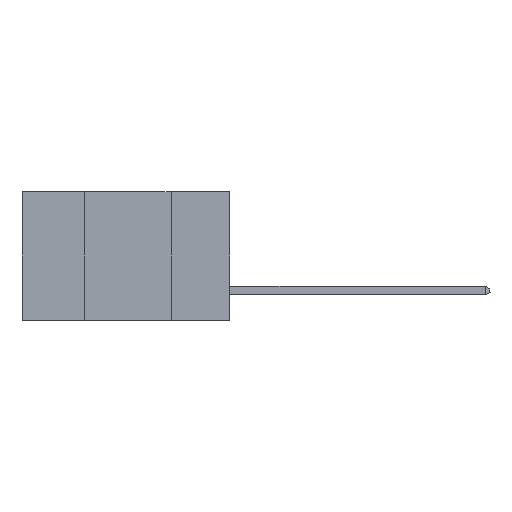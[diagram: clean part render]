
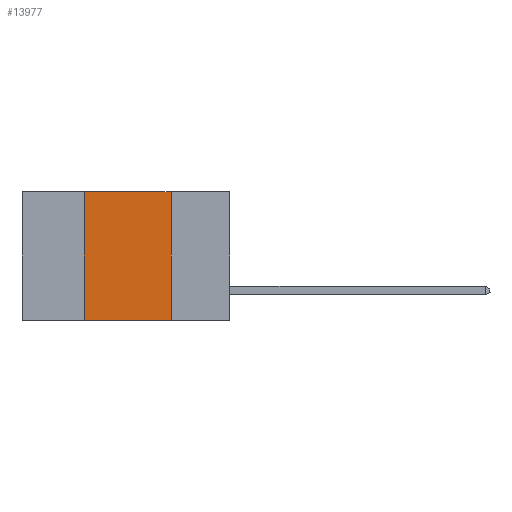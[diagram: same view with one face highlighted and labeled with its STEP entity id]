
A CAD part, left-side view. The second image highlights one B-rep face of the part: STEP entity #13977.
In plain terms, the highlighted planar face has unit normal (-1, 0, 0).
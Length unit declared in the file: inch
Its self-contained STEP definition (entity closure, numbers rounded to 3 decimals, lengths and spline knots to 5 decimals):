
#714 = ORIENTED_EDGE ( 'NONE', *, *, #23727, .T. ) ;
#916 = LINE ( 'NONE', #11618, #8901 ) ;
#1241 = EDGE_CURVE ( 'NONE', #8420, #21967, #916, .T. ) ;
#3220 = AXIS2_PLACEMENT_3D ( 'NONE', #5221, #3767, #10078 ) ;
#3597 = PLANE ( 'NONE',  #3220 ) ;
#3767 = DIRECTION ( 'NONE',  ( 1., 0., 0. ) ) ;
#3939 = ORIENTED_EDGE ( 'NONE', *, *, #4843, .F. ) ;
#4843 = EDGE_CURVE ( 'NONE', #20271, #23851, #8170, .T. ) ;
#5221 = CARTESIAN_POINT ( 'NONE',  ( 0., 0.6, 0. ) ) ;
#7231 = ORIENTED_EDGE ( 'NONE', *, *, #17263, .F. ) ;
#8049 = VECTOR ( 'NONE', #21840, 39.37008 ) ;
#8170 = LINE ( 'NONE', #8718, #8049 ) ;
#8420 = VERTEX_POINT ( 'NONE', #17581 ) ;
#8718 = CARTESIAN_POINT ( 'NONE',  ( 0., 0.17, 0. ) ) ;
#8901 = VECTOR ( 'NONE', #22862, 39.37008 ) ;
#9384 = DIRECTION ( 'NONE',  ( 0., -1., 0. ) ) ;
#10078 = DIRECTION ( 'NONE',  ( 0., 0., -1. ) ) ;
#10566 = ORIENTED_EDGE ( 'NONE', *, *, #1241, .F. ) ;
#10884 = CARTESIAN_POINT ( 'NONE',  ( 0., 0.42, 0. ) ) ;
#11597 = CARTESIAN_POINT ( 'NONE',  ( 0., 0.17, 0. ) ) ;
#11618 = CARTESIAN_POINT ( 'NONE',  ( 0., 0.42, 0. ) ) ;
#12904 = LINE ( 'NONE', #15060, #22272 ) ;
#13977 = ADVANCED_FACE ( 'NONE', ( #14030 ), #3597, .F. ) ;
#14030 = FACE_OUTER_BOUND ( 'NONE', #19481, .T. ) ;
#14361 = CARTESIAN_POINT ( 'NONE',  ( 0., 0.6, -0.37 ) ) ;
#15060 = CARTESIAN_POINT ( 'NONE',  ( 0., 0.6, 0. ) ) ;
#16256 = DIRECTION ( 'NONE',  ( 0., -1., 0. ) ) ;
#17164 = CARTESIAN_POINT ( 'NONE',  ( 0., 0.17, -0.37 ) ) ;
#17263 = EDGE_CURVE ( 'NONE', #21967, #20271, #12904, .T. ) ;
#17581 = CARTESIAN_POINT ( 'NONE',  ( 0., 0.42, -0.37 ) ) ;
#18174 = LINE ( 'NONE', #14361, #19088 ) ;
#19088 = VECTOR ( 'NONE', #16256, 39.37008 ) ;
#19481 = EDGE_LOOP ( 'NONE', ( #3939, #7231, #10566, #714 ) ) ;
#20271 = VERTEX_POINT ( 'NONE', #11597 ) ;
#21840 = DIRECTION ( 'NONE',  ( 0., 0., -1. ) ) ;
#21967 = VERTEX_POINT ( 'NONE', #10884 ) ;
#22272 = VECTOR ( 'NONE', #9384, 39.37008 ) ;
#22862 = DIRECTION ( 'NONE',  ( 0., 0., 1. ) ) ;
#23727 = EDGE_CURVE ( 'NONE', #8420, #23851, #18174, .T. ) ;
#23851 = VERTEX_POINT ( 'NONE', #17164 ) ;
